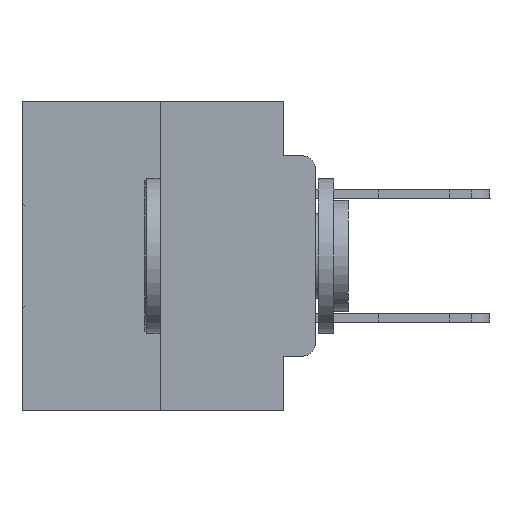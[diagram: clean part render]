
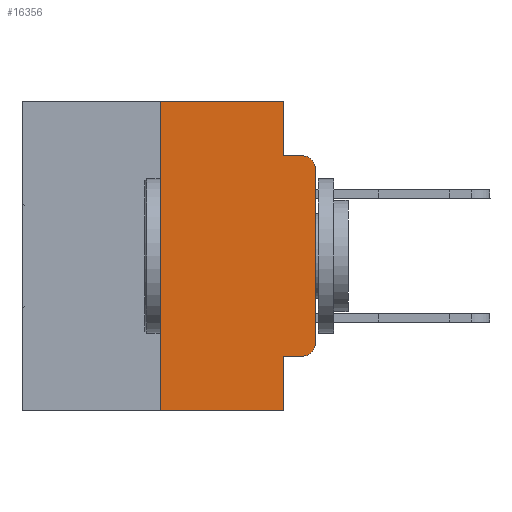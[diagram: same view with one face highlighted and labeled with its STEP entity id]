
A CAD part, left-side view. The second image highlights one B-rep face of the part: STEP entity #16356.
In plain terms, the highlighted planar face has unit normal (-1, 0, 0).
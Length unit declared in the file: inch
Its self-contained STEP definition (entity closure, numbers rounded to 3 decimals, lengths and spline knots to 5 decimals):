
#390 = LINE ( 'NONE', #18585, #18809 ) ;
#586 = CARTESIAN_POINT ( 'NONE',  ( 0., 0.02, -0.4115 ) ) ;
#623 = DIRECTION ( 'NONE',  ( 0., -1., 0. ) ) ;
#1101 = VERTEX_POINT ( 'NONE', #16340 ) ;
#1146 = CIRCLE ( 'NONE', #24686, 0.02 ) ;
#1448 = ORIENTED_EDGE ( 'NONE', *, *, #6585, .T. ) ;
#1499 = DIRECTION ( 'NONE',  ( 0., -1., 0. ) ) ;
#1951 = CARTESIAN_POINT ( 'NONE',  ( 0., 0.051, 0. ) ) ;
#2430 = AXIS2_PLACEMENT_3D ( 'NONE', #11589, #28286, #13994 ) ;
#2506 = ORIENTED_EDGE ( 'NONE', *, *, #14608, .T. ) ;
#2884 = PLANE ( 'NONE',  #29105 ) ;
#3441 = VERTEX_POINT ( 'NONE', #586 ) ;
#3674 = LINE ( 'NONE', #15573, #22743 ) ;
#4963 = EDGE_CURVE ( 'NONE', #3441, #14024, #13003, .T. ) ;
#5240 = VERTEX_POINT ( 'NONE', #19806 ) ;
#6124 = LINE ( 'NONE', #29645, #30818 ) ;
#6240 = LINE ( 'NONE', #17750, #18202 ) ;
#6547 = CARTESIAN_POINT ( 'NONE',  ( 0., 0.25, 0. ) ) ;
#6585 = EDGE_CURVE ( 'NONE', #11490, #3441, #6902, .T. ) ;
#6667 = DIRECTION ( 'NONE',  ( 0., -1., 0. ) ) ;
#6713 = VECTOR ( 'NONE', #20872, 39.37008 ) ;
#6902 = LINE ( 'NONE', #14940, #25240 ) ;
#7881 = CARTESIAN_POINT ( 'NONE',  ( 0., 0.02, -0.1085 ) ) ;
#8170 = DIRECTION ( 'NONE',  ( 0., 0., -1. ) ) ;
#8212 = EDGE_CURVE ( 'NONE', #11490, #30367, #26662, .T. ) ;
#8568 = CARTESIAN_POINT ( 'NONE',  ( 0., 0.051, -0.4115 ) ) ;
#9241 = FACE_OUTER_BOUND ( 'NONE', #20490, .T. ) ;
#9811 = EDGE_CURVE ( 'NONE', #17958, #30045, #13095, .T. ) ;
#10009 = CARTESIAN_POINT ( 'NONE',  ( 0., 0.051, -0.5 ) ) ;
#10285 = DIRECTION ( 'NONE',  ( 0., 0., -1. ) ) ;
#11427 = EDGE_CURVE ( 'NONE', #5240, #1101, #6240, .T. ) ;
#11490 = VERTEX_POINT ( 'NONE', #8568 ) ;
#11589 = CARTESIAN_POINT ( 'NONE',  ( 0., 0.02, -0.3915 ) ) ;
#11878 = ORIENTED_EDGE ( 'NONE', *, *, #11427, .F. ) ;
#12495 = CARTESIAN_POINT ( 'NONE',  ( 0., 0.473, 0. ) ) ;
#12945 = DIRECTION ( 'NONE',  ( 0., 0., 1. ) ) ;
#13003 = CIRCLE ( 'NONE', #2430, 0.02 ) ;
#13007 = EDGE_CURVE ( 'NONE', #1101, #23456, #29706, .T. ) ;
#13095 = LINE ( 'NONE', #6547, #6713 ) ;
#13479 = CARTESIAN_POINT ( 'NONE',  ( 0., 0.051, -0.0885 ) ) ;
#13994 = DIRECTION ( 'NONE',  ( 0., 0., -1. ) ) ;
#14024 = VERTEX_POINT ( 'NONE', #15224 ) ;
#14608 = EDGE_CURVE ( 'NONE', #16128, #23456, #1146, .T. ) ;
#14904 = DIRECTION ( 'NONE',  ( 0., 0., -1. ) ) ;
#14940 = CARTESIAN_POINT ( 'NONE',  ( 0., 0.051, -0.4115 ) ) ;
#15224 = CARTESIAN_POINT ( 'NONE',  ( 0., 0., -0.3915 ) ) ;
#15573 = CARTESIAN_POINT ( 'NONE',  ( 0., 0.473, 0. ) ) ;
#15981 = ORIENTED_EDGE ( 'NONE', *, *, #13007, .F. ) ;
#16128 = VERTEX_POINT ( 'NONE', #16362 ) ;
#16340 = CARTESIAN_POINT ( 'NONE',  ( 0., 0.051, -0.0885 ) ) ;
#16356 = ADVANCED_FACE ( 'NONE', ( #9241 ), #2884, .F. ) ;
#16362 = CARTESIAN_POINT ( 'NONE',  ( 0., 0., -0.1085 ) ) ;
#17750 = CARTESIAN_POINT ( 'NONE',  ( 0., 0.051, 0. ) ) ;
#17798 = EDGE_CURVE ( 'NONE', #14024, #16128, #6124, .T. ) ;
#17958 = VERTEX_POINT ( 'NONE', #24885 ) ;
#18107 = CARTESIAN_POINT ( 'NONE',  ( 0., 0.02, -0.0885 ) ) ;
#18202 = VECTOR ( 'NONE', #8170, 39.37008 ) ;
#18203 = EDGE_CURVE ( 'NONE', #17958, #30367, #390, .T. ) ;
#18585 = CARTESIAN_POINT ( 'NONE',  ( 0., 0.473, -0.5 ) ) ;
#18809 = VECTOR ( 'NONE', #6667, 39.37008 ) ;
#19806 = CARTESIAN_POINT ( 'NONE',  ( 0., 0.051, 0. ) ) ;
#19835 = ORIENTED_EDGE ( 'NONE', *, *, #18203, .T. ) ;
#20324 = VECTOR ( 'NONE', #21112, 39.37008 ) ;
#20490 = EDGE_LOOP ( 'NONE', ( #20839, #2506, #15981, #11878, #26059, #27553, #19835, #26170, #1448, #21339 ) ) ;
#20839 = ORIENTED_EDGE ( 'NONE', *, *, #17798, .T. ) ;
#20872 = DIRECTION ( 'NONE',  ( 0., 0., 1. ) ) ;
#21112 = DIRECTION ( 'NONE',  ( 0., 0., -1. ) ) ;
#21339 = ORIENTED_EDGE ( 'NONE', *, *, #4963, .T. ) ;
#22617 = VECTOR ( 'NONE', #1499, 39.37008 ) ;
#22671 = DIRECTION ( 'NONE',  ( 0., -1., 0. ) ) ;
#22743 = VECTOR ( 'NONE', #22671, 39.37008 ) ;
#22832 = EDGE_CURVE ( 'NONE', #30045, #5240, #3674, .T. ) ;
#23456 = VERTEX_POINT ( 'NONE', #18107 ) ;
#24572 = DIRECTION ( 'NONE',  ( -1., 0., 0. ) ) ;
#24686 = AXIS2_PLACEMENT_3D ( 'NONE', #7881, #24572, #10285 ) ;
#24885 = CARTESIAN_POINT ( 'NONE',  ( 0., 0.25, -0.5 ) ) ;
#25240 = VECTOR ( 'NONE', #623, 39.37008 ) ;
#26059 = ORIENTED_EDGE ( 'NONE', *, *, #22832, .F. ) ;
#26170 = ORIENTED_EDGE ( 'NONE', *, *, #8212, .F. ) ;
#26662 = LINE ( 'NONE', #1951, #20324 ) ;
#27553 = ORIENTED_EDGE ( 'NONE', *, *, #9811, .F. ) ;
#28286 = DIRECTION ( 'NONE',  ( -1., 0., 0. ) ) ;
#29105 = AXIS2_PLACEMENT_3D ( 'NONE', #12495, #29192, #14904 ) ;
#29192 = DIRECTION ( 'NONE',  ( 1., 0., 0. ) ) ;
#29645 = CARTESIAN_POINT ( 'NONE',  ( 0., 0., 0. ) ) ;
#29706 = LINE ( 'NONE', #13479, #22617 ) ;
#30045 = VERTEX_POINT ( 'NONE', #30286 ) ;
#30286 = CARTESIAN_POINT ( 'NONE',  ( 0., 0.25, 0. ) ) ;
#30367 = VERTEX_POINT ( 'NONE', #10009 ) ;
#30818 = VECTOR ( 'NONE', #12945, 39.37008 ) ;
